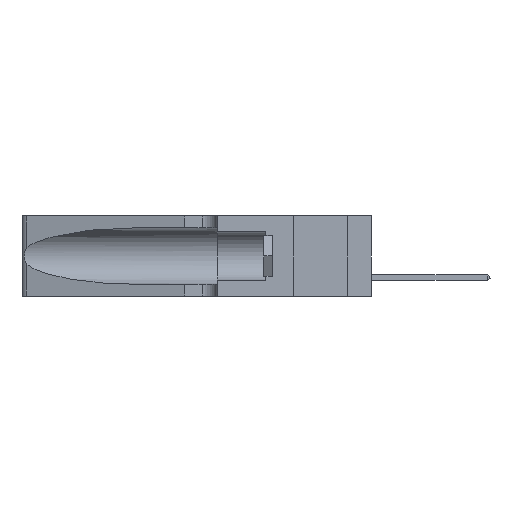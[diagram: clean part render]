
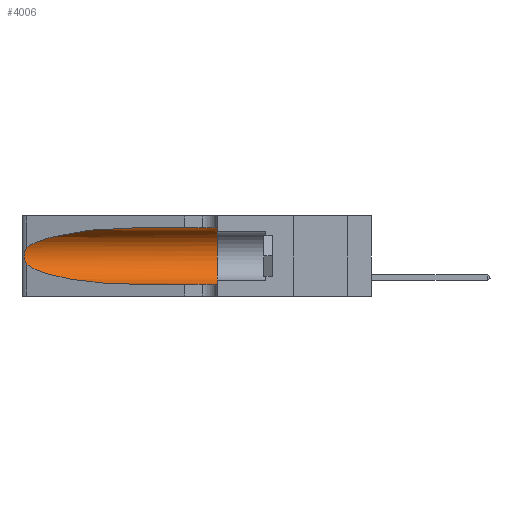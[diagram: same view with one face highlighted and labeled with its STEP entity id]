
A CAD part, left-side view. The second image highlights one B-rep face of the part: STEP entity #4006.
In plain terms, the highlighted cylindrical face has radius 3.308 mm (diameter 6.617 mm), a partial arc.
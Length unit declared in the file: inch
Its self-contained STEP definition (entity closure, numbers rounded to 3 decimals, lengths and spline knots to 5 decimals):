
#166 = CARTESIAN_POINT ( 'NONE',  ( 0.2373, 1.15595, 0.08982 ) ) ;
#453 = VERTEX_POINT ( 'NONE', #16295 ) ;
#1312 = CARTESIAN_POINT ( 'NONE',  ( 0.1305, 0.35, 0.05475 ) ) ;
#1351 = CARTESIAN_POINT ( 'NONE',  ( 0.1305, 0.72297, 0.05475 ) ) ;
#1424 = ORIENTED_EDGE ( 'NONE', *, *, #39399, .F. ) ;
#2493 = CARTESIAN_POINT ( 'NONE',  ( 0.25854, 1.2359, 0.20912 ) ) ;
#3011 =( BOUNDED_CURVE ( )  B_SPLINE_CURVE ( 3, ( #23259, #166, #10202, #13454 ),
 .UNSPECIFIED., .F., .F. ) 
 B_SPLINE_CURVE_WITH_KNOTS ( ( 4, 4 ),
 ( 3.44316, 4.71239 ),
 .UNSPECIFIED. ) 
 CURVE ( )  GEOMETRIC_REPRESENTATION_ITEM ( )  RATIONAL_B_SPLINE_CURVE ( ( 1., 0.87, 0.87, 1. ) ) 
 REPRESENTATION_ITEM ( '' )  );
#3373 = EDGE_CURVE ( 'NONE', #24126, #18533, #38016, .T. ) ;
#3736 = ORIENTED_EDGE ( 'NONE', *, *, #8747, .T. ) ;
#4006 = ADVANCED_FACE ( 'NONE', ( #35463 ), #31431, .F. ) ;
#5085 = CARTESIAN_POINT ( 'NONE',  ( 0.1305, 0.35, 0.31525 ) ) ;
#5435 = CARTESIAN_POINT ( 'NONE',  ( 0.25487, 1.22718, 0.22369 ) ) ;
#7376 = EDGE_CURVE ( 'NONE', #29736, #21146, #21694, .T. ) ;
#8026 = DIRECTION ( 'NONE',  ( 0., 0., 1. ) ) ;
#8690 = CARTESIAN_POINT ( 'NONE',  ( 0.25555, 1.22994, 0.2215 ) ) ;
#8718 = VECTOR ( 'NONE', #39632, 39.37008 ) ;
#8747 = EDGE_CURVE ( 'NONE', #15243, #18533, #33020, .T. ) ;
#9189 = CARTESIAN_POINT ( 'NONE',  ( 0.2373, 1.15595, 0.28018 ) ) ;
#9333 = CARTESIAN_POINT ( 'NONE',  ( 0.25487, 1.22718, 0.22369 ) ) ;
#10202 = CARTESIAN_POINT ( 'NONE',  ( 0.18966, 0.96281, 0.05475 ) ) ;
#11151 = DIRECTION ( 'NONE',  ( 0., -1., 0. ) ) ;
#11650 = CARTESIAN_POINT ( 'NONE',  ( 0.26075, 1.23896, 0.19203 ) ) ;
#11783 = CARTESIAN_POINT ( 'NONE',  ( 0.25555, 1.22993, 0.14849 ) ) ;
#13454 = CARTESIAN_POINT ( 'NONE',  ( 0.1305, 0.72297, 0.05475 ) ) ;
#13536 = VECTOR ( 'NONE', #11151, 39.37008 ) ;
#13702 = CARTESIAN_POINT ( 'NONE',  ( 0.1305, 1.61858, 0.05475 ) ) ;
#14914 = CARTESIAN_POINT ( 'NONE',  ( 0.26017, 1.23833, 0.17102 ) ) ;
#15243 = VERTEX_POINT ( 'NONE', #1351 ) ;
#15433 = AXIS2_PLACEMENT_3D ( 'NONE', #27850, #40864, #8026 ) ;
#16295 = CARTESIAN_POINT ( 'NONE',  ( 0.25487, 1.22718, 0.14631 ) ) ;
#18533 = VERTEX_POINT ( 'NONE', #1312 ) ;
#18689 = CARTESIAN_POINT ( 'NONE',  ( 0.18966, 0.96281, 0.31525 ) ) ;
#19100 = B_SPLINE_CURVE_WITH_KNOTS ( 'NONE', 3,
 ( #5435, #8690, #31081, #41263, #2493, #27969, #11650, #31368, #14914, #31509, #31226, #37745, #11783, #24720 ),
 .UNSPECIFIED., .F., .F.,
 ( 4, 2, 2, 2, 2, 2, 4 ),
 ( 0., 0.00027, 0.00053, 0.00107, 0.0016, 0.00187, 0.00214 ),
 .UNSPECIFIED. ) ;
#20476 = ORIENTED_EDGE ( 'NONE', *, *, #7376, .T. ) ;
#21146 = VERTEX_POINT ( 'NONE', #9333 ) ;
#21368 = ORIENTED_EDGE ( 'NONE', *, *, #28513, .T. ) ;
#21674 = CARTESIAN_POINT ( 'NONE',  ( 0.25487, 1.22718, 0.22369 ) ) ;
#21694 =( BOUNDED_CURVE ( )  B_SPLINE_CURVE ( 3, ( #34815, #18689, #9189, #21674 ),
 .UNSPECIFIED., .F., .T. ) 
 B_SPLINE_CURVE_WITH_KNOTS ( ( 4, 4 ),
 ( 1.5708, 2.84003 ),
 .UNSPECIFIED. ) 
 CURVE ( )  GEOMETRIC_REPRESENTATION_ITEM ( )  RATIONAL_B_SPLINE_CURVE ( ( 1., 0.87, 0.87, 1. ) ) 
 REPRESENTATION_ITEM ( '' )  );
#23259 = CARTESIAN_POINT ( 'NONE',  ( 0.25487, 1.22718, 0.14631 ) ) ;
#23994 = ORIENTED_EDGE ( 'NONE', *, *, #3373, .F. ) ;
#24126 = VERTEX_POINT ( 'NONE', #5085 ) ;
#24720 = CARTESIAN_POINT ( 'NONE',  ( 0.25487, 1.22718, 0.14631 ) ) ;
#27850 = CARTESIAN_POINT ( 'NONE',  ( 0.1305, 0.35, 0.185 ) ) ;
#27969 = CARTESIAN_POINT ( 'NONE',  ( 0.26018, 1.23835, 0.19895 ) ) ;
#28513 = EDGE_CURVE ( 'NONE', #453, #15243, #3011, .T. ) ;
#28783 = DIRECTION ( 'NONE',  ( 0., -1., 0. ) ) ;
#29736 = VERTEX_POINT ( 'NONE', #33257 ) ;
#30343 = LINE ( 'NONE', #40082, #13536 ) ;
#31081 = CARTESIAN_POINT ( 'NONE',  ( 0.25639, 1.23184, 0.21858 ) ) ;
#31226 = CARTESIAN_POINT ( 'NONE',  ( 0.25789, 1.23486, 0.15765 ) ) ;
#31368 = CARTESIAN_POINT ( 'NONE',  ( 0.26075, 1.23896, 0.178 ) ) ;
#31431 = CYLINDRICAL_SURFACE ( 'NONE', #40666, 0.13025 ) ;
#31509 = CARTESIAN_POINT ( 'NONE',  ( 0.25856, 1.23593, 0.16098 ) ) ;
#31882 = CARTESIAN_POINT ( 'NONE',  ( 0.1305, 1.61858, 0.185 ) ) ;
#33020 = LINE ( 'NONE', #13702, #8718 ) ;
#33257 = CARTESIAN_POINT ( 'NONE',  ( 0.1305, 0.72297, 0.31525 ) ) ;
#33334 = EDGE_LOOP ( 'NONE', ( #20476, #41971, #21368, #3736, #23994, #1424 ) ) ;
#34815 = CARTESIAN_POINT ( 'NONE',  ( 0.1305, 0.72297, 0.31525 ) ) ;
#35111 = DIRECTION ( 'NONE',  ( 0., 0., -1. ) ) ;
#35463 = FACE_OUTER_BOUND ( 'NONE', #33334, .T. ) ;
#36325 = EDGE_CURVE ( 'NONE', #21146, #453, #19100, .T. ) ;
#37745 = CARTESIAN_POINT ( 'NONE',  ( 0.25639, 1.23186, 0.15144 ) ) ;
#38016 = CIRCLE ( 'NONE', #15433, 0.13025 ) ;
#39399 = EDGE_CURVE ( 'NONE', #29736, #24126, #30343, .T. ) ;
#39632 = DIRECTION ( 'NONE',  ( 0., -1., 0. ) ) ;
#40082 = CARTESIAN_POINT ( 'NONE',  ( 0.1305, 1.61858, 0.31525 ) ) ;
#40666 = AXIS2_PLACEMENT_3D ( 'NONE', #31882, #28783, #35111 ) ;
#40864 = DIRECTION ( 'NONE',  ( 0., 1., 0. ) ) ;
#41263 = CARTESIAN_POINT ( 'NONE',  ( 0.25787, 1.23484, 0.2124 ) ) ;
#41971 = ORIENTED_EDGE ( 'NONE', *, *, #36325, .T. ) ;
